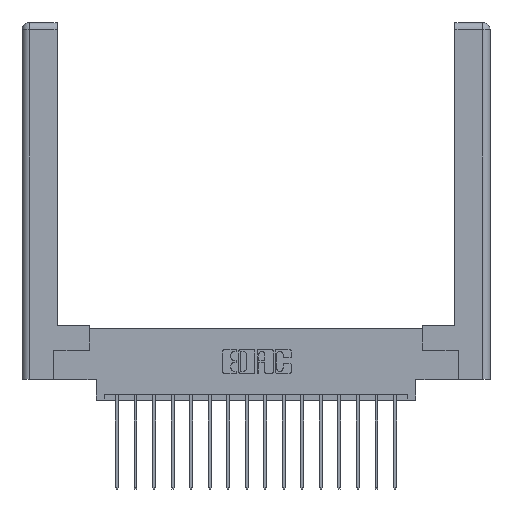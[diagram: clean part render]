
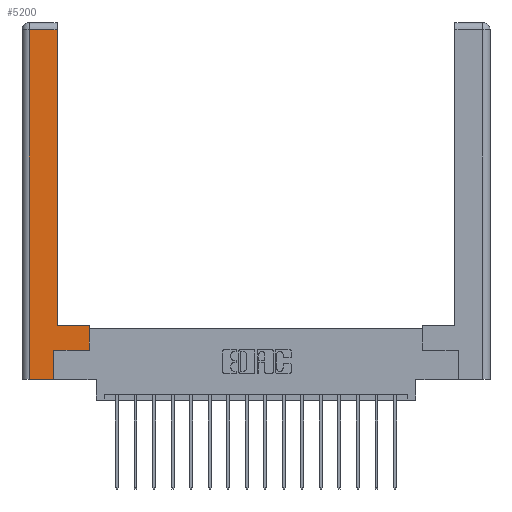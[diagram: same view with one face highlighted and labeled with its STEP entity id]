
A CAD part, top view. The second image highlights one B-rep face of the part: STEP entity #5200.
In plain terms, the highlighted planar face has unit normal (0, 0, 1).
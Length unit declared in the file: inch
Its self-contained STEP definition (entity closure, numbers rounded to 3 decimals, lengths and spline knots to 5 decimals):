
#30 = DIRECTION ( 'NONE',  ( -1., 0., 0. ) ) ;
#518 = ORIENTED_EDGE ( 'NONE', *, *, #14763, .T. ) ;
#1874 = EDGE_CURVE ( 'NONE', #12983, #17349, #2797, .T. ) ;
#2340 = VECTOR ( 'NONE', #7042, 39.37008 ) ;
#2797 = LINE ( 'NONE', #3344, #9731 ) ;
#2798 = LINE ( 'NONE', #11075, #2340 ) ;
#2839 = CARTESIAN_POINT ( 'NONE',  ( 0.565, 0.45, 0. ) ) ;
#3134 = VERTEX_POINT ( 'NONE', #2839 ) ;
#3200 = EDGE_CURVE ( 'NONE', #10255, #11720, #14854, .T. ) ;
#3344 = CARTESIAN_POINT ( 'NONE',  ( 0.265, 0., 0. ) ) ;
#3391 = ORIENTED_EDGE ( 'NONE', *, *, #3200, .T. ) ;
#3486 = VECTOR ( 'NONE', #7271, 39.37008 ) ;
#3590 = VECTOR ( 'NONE', #8670, 39.37008 ) ;
#3951 = CARTESIAN_POINT ( 'NONE',  ( 0., 0., 0. ) ) ;
#4315 = ORIENTED_EDGE ( 'NONE', *, *, #12460, .T. ) ;
#4542 = ORIENTED_EDGE ( 'NONE', *, *, #8986, .T. ) ;
#4766 = VERTEX_POINT ( 'NONE', #14193 ) ;
#4824 = ORIENTED_EDGE ( 'NONE', *, *, #14093, .T. ) ;
#5142 = LINE ( 'NONE', #11019, #11175 ) ;
#5200 = ADVANCED_FACE ( 'NONE', ( #10525 ), #13796, .F. ) ;
#6501 = ORIENTED_EDGE ( 'NONE', *, *, #1874, .T. ) ;
#6568 = EDGE_CURVE ( 'NONE', #7927, #15946, #7299, .T. ) ;
#7004 = CARTESIAN_POINT ( 'NONE',  ( 0.265, 0., 0. ) ) ;
#7042 = DIRECTION ( 'NONE',  ( 0., -1., 0. ) ) ;
#7271 = DIRECTION ( 'NONE',  ( 0., 1., 0. ) ) ;
#7299 = LINE ( 'NONE', #17163, #3486 ) ;
#7927 = VERTEX_POINT ( 'NONE', #18092 ) ;
#8274 = DIRECTION ( 'NONE',  ( 0., 0., -1. ) ) ;
#8346 = LINE ( 'NONE', #11555, #8571 ) ;
#8571 = VECTOR ( 'NONE', #30, 39.37008 ) ;
#8670 = DIRECTION ( 'NONE',  ( 1., 0., 0. ) ) ;
#8815 = EDGE_LOOP ( 'NONE', ( #13013, #4542, #518, #6501, #4315, #3391, #4824, #11081 ) ) ;
#8986 = EDGE_CURVE ( 'NONE', #15946, #4766, #13056, .T. ) ;
#9231 = VECTOR ( 'NONE', #16710, 39.37008 ) ;
#9731 = VECTOR ( 'NONE', #10897, 39.37008 ) ;
#10255 = VERTEX_POINT ( 'NONE', #18149 ) ;
#10525 = FACE_OUTER_BOUND ( 'NONE', #8815, .T. ) ;
#10743 = EDGE_CURVE ( 'NONE', #3134, #7927, #8346, .T. ) ;
#10897 = DIRECTION ( 'NONE',  ( 1., 0., 0. ) ) ;
#10958 = CARTESIAN_POINT ( 'NONE',  ( 0.0615, 0., 0. ) ) ;
#11019 = CARTESIAN_POINT ( 'NONE',  ( 0.265, 0.245, 0. ) ) ;
#11075 = CARTESIAN_POINT ( 'NONE',  ( 0.0615, 0., 0. ) ) ;
#11081 = ORIENTED_EDGE ( 'NONE', *, *, #10743, .T. ) ;
#11087 = CARTESIAN_POINT ( 'NONE',  ( 0.295, 2.94, 0. ) ) ;
#11175 = VECTOR ( 'NONE', #18359, 39.37008 ) ;
#11555 = CARTESIAN_POINT ( 'NONE',  ( 0.295, 0.45, 0. ) ) ;
#11720 = VERTEX_POINT ( 'NONE', #12207 ) ;
#12207 = CARTESIAN_POINT ( 'NONE',  ( 0.565, 0.245, 0. ) ) ;
#12460 = EDGE_CURVE ( 'NONE', #17349, #10255, #5142, .T. ) ;
#12983 = VERTEX_POINT ( 'NONE', #10958 ) ;
#13013 = ORIENTED_EDGE ( 'NONE', *, *, #6568, .T. ) ;
#13056 = LINE ( 'NONE', #15287, #9231 ) ;
#13796 = PLANE ( 'NONE',  #13815 ) ;
#13810 = VECTOR ( 'NONE', #13858, 39.37008 ) ;
#13815 = AXIS2_PLACEMENT_3D ( 'NONE', #3951, #8274, #17445 ) ;
#13858 = DIRECTION ( 'NONE',  ( 0., 1., 0. ) ) ;
#14093 = EDGE_CURVE ( 'NONE', #11720, #3134, #14511, .T. ) ;
#14193 = CARTESIAN_POINT ( 'NONE',  ( 0.0615, 2.94, 0. ) ) ;
#14511 = LINE ( 'NONE', #18198, #13810 ) ;
#14763 = EDGE_CURVE ( 'NONE', #4766, #12983, #2798, .T. ) ;
#14854 = LINE ( 'NONE', #15766, #3590 ) ;
#15287 = CARTESIAN_POINT ( 'NONE',  ( 0.0615, 2.94, 0. ) ) ;
#15766 = CARTESIAN_POINT ( 'NONE',  ( 0.565, 0.245, 0. ) ) ;
#15946 = VERTEX_POINT ( 'NONE', #11087 ) ;
#16710 = DIRECTION ( 'NONE',  ( -1., 0., 0. ) ) ;
#17163 = CARTESIAN_POINT ( 'NONE',  ( 0.295, 3., 0. ) ) ;
#17349 = VERTEX_POINT ( 'NONE', #7004 ) ;
#17445 = DIRECTION ( 'NONE',  ( -1., 0., 0. ) ) ;
#18092 = CARTESIAN_POINT ( 'NONE',  ( 0.295, 0.45, 0. ) ) ;
#18149 = CARTESIAN_POINT ( 'NONE',  ( 0.265, 0.245, 0. ) ) ;
#18198 = CARTESIAN_POINT ( 'NONE',  ( 0.565, 0.45, 0. ) ) ;
#18359 = DIRECTION ( 'NONE',  ( 0., 1., 0. ) ) ;
